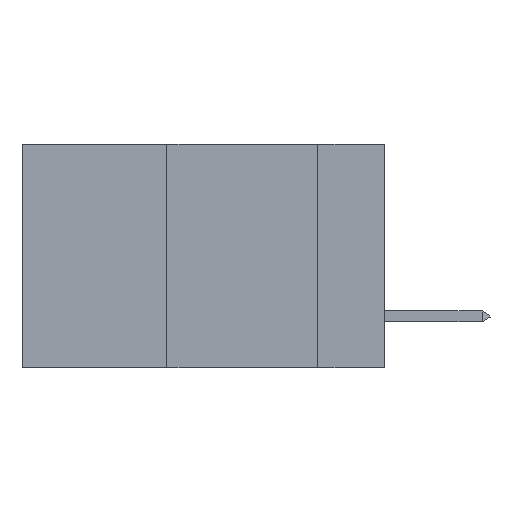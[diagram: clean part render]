
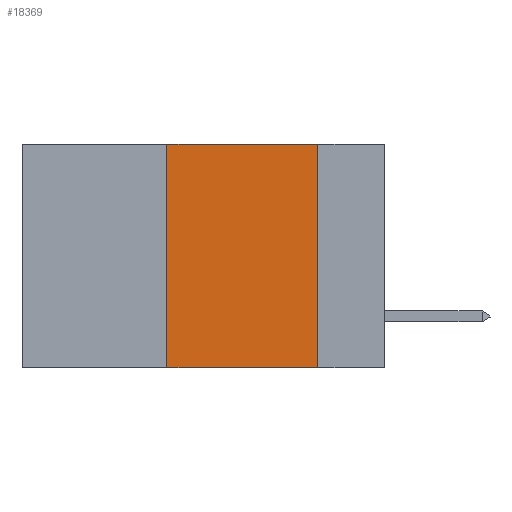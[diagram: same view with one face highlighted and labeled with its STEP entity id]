
A CAD part, left-side view. The second image highlights one B-rep face of the part: STEP entity #18369.
In plain terms, the highlighted planar face has unit normal (-1, 0, 0).
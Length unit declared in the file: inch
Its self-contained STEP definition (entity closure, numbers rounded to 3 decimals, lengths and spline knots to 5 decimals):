
#116 = CARTESIAN_POINT ( 'NONE',  ( 0., 0.11, 0. ) ) ;
#635 = CARTESIAN_POINT ( 'NONE',  ( 0., 0.6, 0. ) ) ;
#1343 = EDGE_CURVE ( 'NONE', #4270, #13694, #18603, .T. ) ;
#1362 = DIRECTION ( 'NONE',  ( 0., -1., 0. ) ) ;
#2353 = CARTESIAN_POINT ( 'NONE',  ( 0., 0.6, -0.37 ) ) ;
#2579 = LINE ( 'NONE', #8013, #7546 ) ;
#2959 = DIRECTION ( 'NONE',  ( 0., 0., -1. ) ) ;
#3099 = VECTOR ( 'NONE', #14784, 39.37008 ) ;
#4270 = VERTEX_POINT ( 'NONE', #16413 ) ;
#4561 = LINE ( 'NONE', #635, #19382 ) ;
#4673 = FACE_OUTER_BOUND ( 'NONE', #13744, .T. ) ;
#4870 = ORIENTED_EDGE ( 'NONE', *, *, #1343, .T. ) ;
#5027 = AXIS2_PLACEMENT_3D ( 'NONE', #8980, #19475, #2959 ) ;
#5757 = PLANE ( 'NONE',  #5027 ) ;
#5958 = LINE ( 'NONE', #18949, #3099 ) ;
#6728 = DIRECTION ( 'NONE',  ( 0., -1., 0. ) ) ;
#6989 = EDGE_CURVE ( 'NONE', #11320, #18988, #4561, .T. ) ;
#7546 = VECTOR ( 'NONE', #9392, 39.37008 ) ;
#8013 = CARTESIAN_POINT ( 'NONE',  ( 0., 0.11, 0. ) ) ;
#8298 = CARTESIAN_POINT ( 'NONE',  ( 0., 0.36, 0. ) ) ;
#8427 = EDGE_CURVE ( 'NONE', #18988, #13694, #2579, .T. ) ;
#8980 = CARTESIAN_POINT ( 'NONE',  ( 0., 0.6, 0. ) ) ;
#9392 = DIRECTION ( 'NONE',  ( 0., 0., -1. ) ) ;
#11211 = ORIENTED_EDGE ( 'NONE', *, *, #6989, .F. ) ;
#11320 = VERTEX_POINT ( 'NONE', #8298 ) ;
#11618 = VECTOR ( 'NONE', #1362, 39.37008 ) ;
#12257 = CARTESIAN_POINT ( 'NONE',  ( 0., 0.11, -0.37 ) ) ;
#12548 = ORIENTED_EDGE ( 'NONE', *, *, #8427, .F. ) ;
#13694 = VERTEX_POINT ( 'NONE', #12257 ) ;
#13744 = EDGE_LOOP ( 'NONE', ( #12548, #11211, #15223, #4870 ) ) ;
#14784 = DIRECTION ( 'NONE',  ( 0., 0., 1. ) ) ;
#15223 = ORIENTED_EDGE ( 'NONE', *, *, #16021, .F. ) ;
#16021 = EDGE_CURVE ( 'NONE', #4270, #11320, #5958, .T. ) ;
#16413 = CARTESIAN_POINT ( 'NONE',  ( 0., 0.36, -0.37 ) ) ;
#18369 = ADVANCED_FACE ( 'NONE', ( #4673 ), #5757, .F. ) ;
#18603 = LINE ( 'NONE', #2353, #11618 ) ;
#18949 = CARTESIAN_POINT ( 'NONE',  ( 0., 0.36, 0. ) ) ;
#18988 = VERTEX_POINT ( 'NONE', #116 ) ;
#19382 = VECTOR ( 'NONE', #6728, 39.37008 ) ;
#19475 = DIRECTION ( 'NONE',  ( 1., 0., 0. ) ) ;
